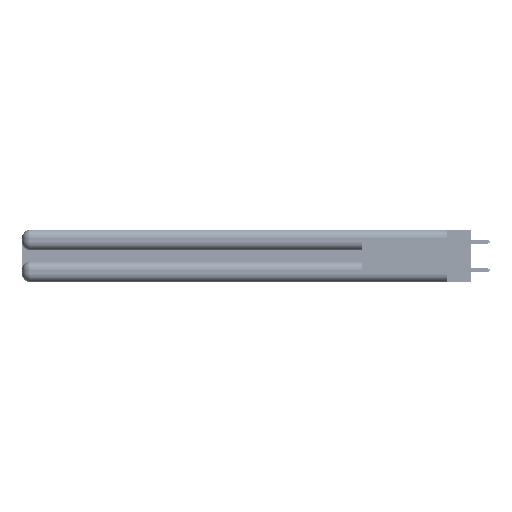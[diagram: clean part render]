
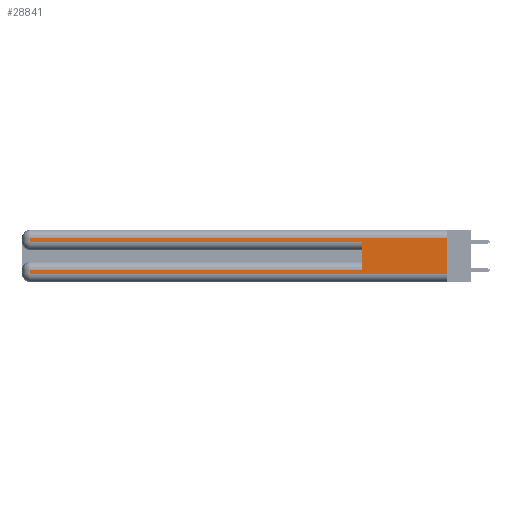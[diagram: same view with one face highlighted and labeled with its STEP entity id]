
A CAD part, left-side view. The second image highlights one B-rep face of the part: STEP entity #28841.
In plain terms, the highlighted planar face has unit normal (-1, 0, 0).
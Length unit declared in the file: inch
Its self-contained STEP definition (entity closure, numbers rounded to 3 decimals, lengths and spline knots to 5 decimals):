
#52 = VERTEX_POINT ( 'NONE', #25695 ) ;
#746 = VECTOR ( 'NONE', #7775, 39.37008 ) ;
#794 = VECTOR ( 'NONE', #12125, 39.37008 ) ;
#824 = CARTESIAN_POINT ( 'NONE',  ( 0., 0., 0.31 ) ) ;
#1986 = ORIENTED_EDGE ( 'NONE', *, *, #48472, .T. ) ;
#4645 = LINE ( 'NONE', #824, #8071 ) ;
#5048 = VECTOR ( 'NONE', #27034, 39.37008 ) ;
#5857 = VERTEX_POINT ( 'NONE', #44860 ) ;
#7233 = ORIENTED_EDGE ( 'NONE', *, *, #19704, .T. ) ;
#7775 = DIRECTION ( 'NONE',  ( 0., 0., -1. ) ) ;
#7898 = CARTESIAN_POINT ( 'NONE',  ( 0., 0.6, 0.145 ) ) ;
#8071 = VECTOR ( 'NONE', #18364, 39.37008 ) ;
#8345 = EDGE_LOOP ( 'NONE', ( #13821, #1986, #54591, #7233, #31554, #37231, #17778, #34585 ) ) ;
#10718 = VECTOR ( 'NONE', #43572, 39.37008 ) ;
#12125 = DIRECTION ( 'NONE',  ( 0., 1., 0. ) ) ;
#12203 = CARTESIAN_POINT ( 'NONE',  ( 0., 0., 0.37 ) ) ;
#12339 = DIRECTION ( 'NONE',  ( 0., 0., 1. ) ) ;
#12548 = FACE_OUTER_BOUND ( 'NONE', #8345, .T. ) ;
#12654 = CARTESIAN_POINT ( 'NONE',  ( 0., 2.94, 0.37 ) ) ;
#13534 = VECTOR ( 'NONE', #46215, 39.37008 ) ;
#13821 = ORIENTED_EDGE ( 'NONE', *, *, #44566, .F. ) ;
#14787 = VECTOR ( 'NONE', #12339, 39.37008 ) ;
#15243 = EDGE_CURVE ( 'NONE', #46842, #21450, #16843, .T. ) ;
#15564 = LINE ( 'NONE', #12654, #10718 ) ;
#15931 = CARTESIAN_POINT ( 'NONE',  ( 0., 0., 0.37 ) ) ;
#16843 = LINE ( 'NONE', #7898, #14787 ) ;
#17778 = ORIENTED_EDGE ( 'NONE', *, *, #18286, .T. ) ;
#17807 = CARTESIAN_POINT ( 'NONE',  ( 0., 0.6, 0.085 ) ) ;
#18286 = EDGE_CURVE ( 'NONE', #21597, #52, #27115, .T. ) ;
#18364 = DIRECTION ( 'NONE',  ( 0., 1., 0. ) ) ;
#19704 = EDGE_CURVE ( 'NONE', #28968, #21450, #48821, .T. ) ;
#21450 = VERTEX_POINT ( 'NONE', #41221 ) ;
#21597 = VERTEX_POINT ( 'NONE', #41975 ) ;
#22466 = EDGE_CURVE ( 'NONE', #52, #52998, #30563, .T. ) ;
#23637 = VECTOR ( 'NONE', #51947, 39.37008 ) ;
#23887 = CARTESIAN_POINT ( 'NONE',  ( 0., 2.94, 0.31 ) ) ;
#25695 = CARTESIAN_POINT ( 'NONE',  ( 0., 2.94, 0.06 ) ) ;
#26651 = CARTESIAN_POINT ( 'NONE',  ( 0., 0., 0.06 ) ) ;
#27034 = DIRECTION ( 'NONE',  ( 0., -1., 0. ) ) ;
#27115 = LINE ( 'NONE', #38238, #23637 ) ;
#28841 = ADVANCED_FACE ( 'NONE', ( #12548 ), #55859, .F. ) ;
#28968 = VERTEX_POINT ( 'NONE', #47804 ) ;
#29236 = DIRECTION ( 'NONE',  ( 1., 0., 0. ) ) ;
#29428 = DIRECTION ( 'NONE',  ( 0., 0., -1. ) ) ;
#30563 = LINE ( 'NONE', #26651, #5048 ) ;
#31554 = ORIENTED_EDGE ( 'NONE', *, *, #15243, .F. ) ;
#32109 = CARTESIAN_POINT ( 'NONE',  ( 0., 0., 0.285 ) ) ;
#34511 = CARTESIAN_POINT ( 'NONE',  ( 0., 0., 0.06 ) ) ;
#34585 = ORIENTED_EDGE ( 'NONE', *, *, #22466, .T. ) ;
#36422 = VERTEX_POINT ( 'NONE', #23887 ) ;
#37231 = ORIENTED_EDGE ( 'NONE', *, *, #54582, .T. ) ;
#38238 = CARTESIAN_POINT ( 'NONE',  ( 0., 2.94, 0.37 ) ) ;
#41221 = CARTESIAN_POINT ( 'NONE',  ( 0., 0.6, 0.285 ) ) ;
#41975 = CARTESIAN_POINT ( 'NONE',  ( 0., 2.94, 0.085 ) ) ;
#42894 = LINE ( 'NONE', #12203, #746 ) ;
#43572 = DIRECTION ( 'NONE',  ( 0., 0., -1. ) ) ;
#44566 = EDGE_CURVE ( 'NONE', #5857, #52998, #42894, .T. ) ;
#44860 = CARTESIAN_POINT ( 'NONE',  ( 0., 0., 0.31 ) ) ;
#46215 = DIRECTION ( 'NONE',  ( 0., -1., 0. ) ) ;
#46842 = VERTEX_POINT ( 'NONE', #17807 ) ;
#47804 = CARTESIAN_POINT ( 'NONE',  ( 0., 2.94, 0.285 ) ) ;
#47932 = AXIS2_PLACEMENT_3D ( 'NONE', #15931, #29236, #29428 ) ;
#48472 = EDGE_CURVE ( 'NONE', #5857, #36422, #4645, .T. ) ;
#48821 = LINE ( 'NONE', #32109, #13534 ) ;
#49415 = EDGE_CURVE ( 'NONE', #36422, #28968, #15564, .T. ) ;
#51348 = CARTESIAN_POINT ( 'NONE',  ( 0., 0., 0.085 ) ) ;
#51947 = DIRECTION ( 'NONE',  ( 0., 0., -1. ) ) ;
#52998 = VERTEX_POINT ( 'NONE', #34511 ) ;
#54582 = EDGE_CURVE ( 'NONE', #46842, #21597, #56713, .T. ) ;
#54591 = ORIENTED_EDGE ( 'NONE', *, *, #49415, .T. ) ;
#55859 = PLANE ( 'NONE',  #47932 ) ;
#56713 = LINE ( 'NONE', #51348, #794 ) ;
